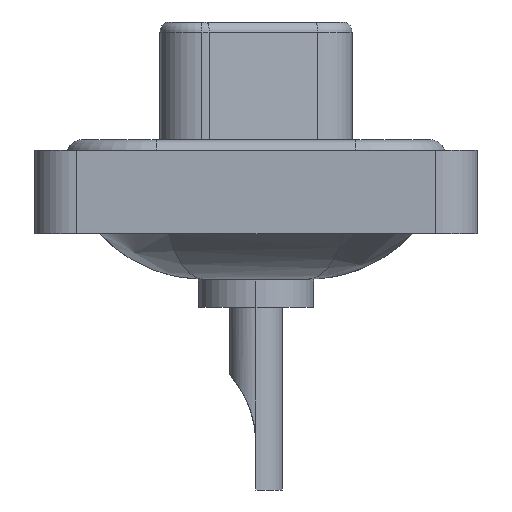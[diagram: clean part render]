
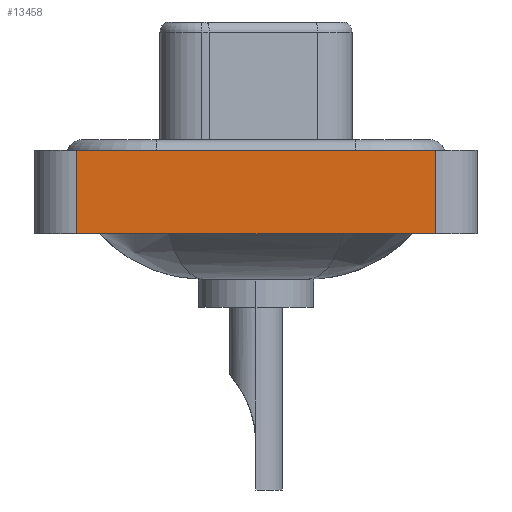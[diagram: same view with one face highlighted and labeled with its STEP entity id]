
A CAD part, left-side view. The second image highlights one B-rep face of the part: STEP entity #13458.
In plain terms, the highlighted planar face has unit normal (-1, 0, 0).
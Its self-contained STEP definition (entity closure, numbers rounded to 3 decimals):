
#522 = ORIENTED_EDGE ( 'NONE', *, *, #9459, .T. ) ;
#1734 = ORIENTED_EDGE ( 'NONE', *, *, #8264, .F. ) ;
#2733 = CARTESIAN_POINT ( 'NONE',  ( -7.3, 8.55, -3.6 ) ) ;
#4154 = VECTOR ( 'NONE', #11900, 1000. ) ;
#4195 = EDGE_CURVE ( 'NONE', #7333, #10822, #8537, .T. ) ;
#4607 = DIRECTION ( 'NONE',  ( 0., 0., 1. ) ) ;
#5172 = DIRECTION ( 'NONE',  ( -1., 0., 0. ) ) ;
#5274 = CARTESIAN_POINT ( 'NONE',  ( -7.3, -8.55, -3.6 ) ) ;
#5412 = CARTESIAN_POINT ( 'NONE',  ( -7.3, 8.55, 0.4 ) ) ;
#5491 = VERTEX_POINT ( 'NONE', #5541 ) ;
#5541 = CARTESIAN_POINT ( 'NONE',  ( -7.3, -8.55, -3.6 ) ) ;
#5768 = LINE ( 'NONE', #2733, #4154 ) ;
#6536 = CARTESIAN_POINT ( 'NONE',  ( -7.3, -8.55, 0.4 ) ) ;
#6808 = AXIS2_PLACEMENT_3D ( 'NONE', #5274, #5172, #11410 ) ;
#7333 = VERTEX_POINT ( 'NONE', #5412 ) ;
#7468 = CARTESIAN_POINT ( 'NONE',  ( -7.3, -8.55, -3.6 ) ) ;
#8264 = EDGE_CURVE ( 'NONE', #13305, #7333, #5768, .T. ) ;
#8370 = VECTOR ( 'NONE', #17940, 1000. ) ;
#8537 = LINE ( 'NONE', #14434, #18942 ) ;
#9459 = EDGE_CURVE ( 'NONE', #5491, #10822, #17976, .T. ) ;
#10822 = VERTEX_POINT ( 'NONE', #6536 ) ;
#11410 = DIRECTION ( 'NONE',  ( 0., 0., 1. ) ) ;
#11511 = PLANE ( 'NONE',  #6808 ) ;
#11900 = DIRECTION ( 'NONE',  ( 0., 0., 1. ) ) ;
#12215 = CARTESIAN_POINT ( 'NONE',  ( -7.3, 8.55, -3.6 ) ) ;
#12878 = EDGE_LOOP ( 'NONE', ( #522, #18739, #1734, #17197 ) ) ;
#13305 = VERTEX_POINT ( 'NONE', #12215 ) ;
#13458 = ADVANCED_FACE ( 'NONE', ( #18925 ), #11511, .T. ) ;
#14434 = CARTESIAN_POINT ( 'NONE',  ( -7.3, -8.55, 0.4 ) ) ;
#14543 = DIRECTION ( 'NONE',  ( 0., -1., 0. ) ) ;
#14638 = LINE ( 'NONE', #17844, #8370 ) ;
#15001 = EDGE_CURVE ( 'NONE', #13305, #5491, #14638, .T. ) ;
#16754 = VECTOR ( 'NONE', #4607, 1000. ) ;
#17197 = ORIENTED_EDGE ( 'NONE', *, *, #15001, .T. ) ;
#17844 = CARTESIAN_POINT ( 'NONE',  ( -7.3, -8.55, -3.6 ) ) ;
#17940 = DIRECTION ( 'NONE',  ( 0., -1., 0. ) ) ;
#17976 = LINE ( 'NONE', #7468, #16754 ) ;
#18739 = ORIENTED_EDGE ( 'NONE', *, *, #4195, .F. ) ;
#18925 = FACE_OUTER_BOUND ( 'NONE', #12878, .T. ) ;
#18942 = VECTOR ( 'NONE', #14543, 1000. ) ;
